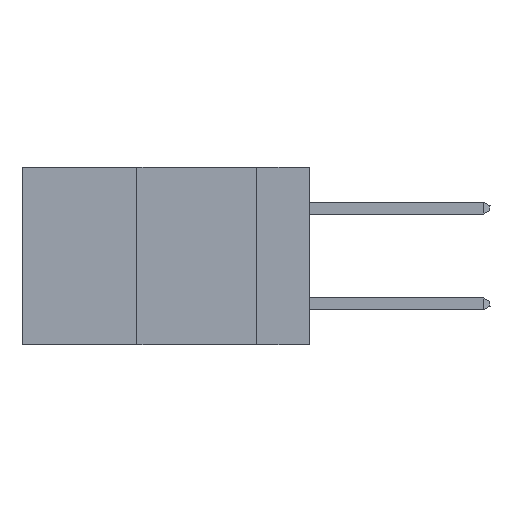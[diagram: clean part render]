
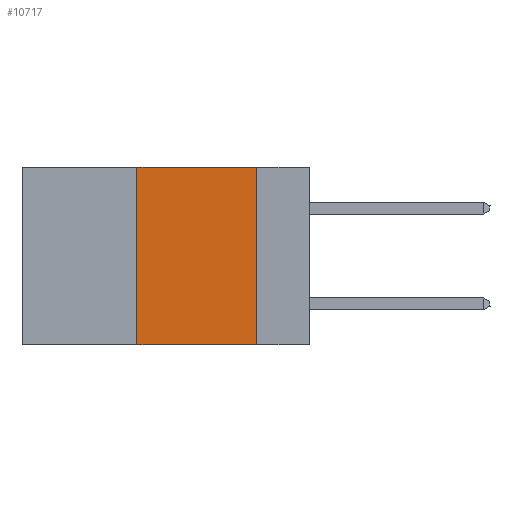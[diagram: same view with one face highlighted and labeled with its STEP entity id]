
A CAD part, left-side view. The second image highlights one B-rep face of the part: STEP entity #10717.
In plain terms, the highlighted planar face has unit normal (-1, 0, 0).
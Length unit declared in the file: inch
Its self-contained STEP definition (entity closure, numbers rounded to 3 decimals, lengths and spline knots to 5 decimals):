
#1146 = CARTESIAN_POINT ( 'NONE',  ( 0., 0.11, 0. ) ) ;
#1238 = VERTEX_POINT ( 'NONE', #8673 ) ;
#1321 = CARTESIAN_POINT ( 'NONE',  ( 0., 0.6, -0.37 ) ) ;
#1409 = VERTEX_POINT ( 'NONE', #10183 ) ;
#2096 = DIRECTION ( 'NONE',  ( 1., 0., 0. ) ) ;
#2197 = CARTESIAN_POINT ( 'NONE',  ( 0., 0.36, 0. ) ) ;
#2538 = ORIENTED_EDGE ( 'NONE', *, *, #3859, .F. ) ;
#2765 = FACE_OUTER_BOUND ( 'NONE', #9838, .T. ) ;
#2970 = CARTESIAN_POINT ( 'NONE',  ( 0., 0.6, 0. ) ) ;
#3279 = DIRECTION ( 'NONE',  ( 0., -1., 0. ) ) ;
#3540 = CARTESIAN_POINT ( 'NONE',  ( 0., 0.36, -0.37 ) ) ;
#3859 = EDGE_CURVE ( 'NONE', #5016, #6405, #11107, .T. ) ;
#4099 = ORIENTED_EDGE ( 'NONE', *, *, #12508, .T. ) ;
#4208 = DIRECTION ( 'NONE',  ( 0., 0., -1. ) ) ;
#4280 = LINE ( 'NONE', #1321, #11281 ) ;
#4393 = VECTOR ( 'NONE', #7071, 39.37008 ) ;
#4501 = EDGE_CURVE ( 'NONE', #6405, #1409, #8302, .T. ) ;
#4865 = VECTOR ( 'NONE', #5675, 39.37008 ) ;
#5016 = VERTEX_POINT ( 'NONE', #3540 ) ;
#5675 = DIRECTION ( 'NONE',  ( 0., 0., 1. ) ) ;
#6405 = VERTEX_POINT ( 'NONE', #2197 ) ;
#7071 = DIRECTION ( 'NONE',  ( 0., -1., 0. ) ) ;
#7522 = LINE ( 'NONE', #1146, #12227 ) ;
#7908 = DIRECTION ( 'NONE',  ( 0., 0., -1. ) ) ;
#8046 = PLANE ( 'NONE',  #8384 ) ;
#8076 = CARTESIAN_POINT ( 'NONE',  ( 0., 0.6, 0. ) ) ;
#8287 = ORIENTED_EDGE ( 'NONE', *, *, #12796, .F. ) ;
#8302 = LINE ( 'NONE', #8076, #4393 ) ;
#8384 = AXIS2_PLACEMENT_3D ( 'NONE', #2970, #2096, #7908 ) ;
#8673 = CARTESIAN_POINT ( 'NONE',  ( 0., 0.11, -0.37 ) ) ;
#9650 = CARTESIAN_POINT ( 'NONE',  ( 0., 0.36, 0. ) ) ;
#9838 = EDGE_LOOP ( 'NONE', ( #8287, #11392, #2538, #4099 ) ) ;
#10183 = CARTESIAN_POINT ( 'NONE',  ( 0., 0.11, 0. ) ) ;
#10717 = ADVANCED_FACE ( 'NONE', ( #2765 ), #8046, .F. ) ;
#11107 = LINE ( 'NONE', #9650, #4865 ) ;
#11281 = VECTOR ( 'NONE', #3279, 39.37008 ) ;
#11392 = ORIENTED_EDGE ( 'NONE', *, *, #4501, .F. ) ;
#12227 = VECTOR ( 'NONE', #4208, 39.37008 ) ;
#12508 = EDGE_CURVE ( 'NONE', #5016, #1238, #4280, .T. ) ;
#12796 = EDGE_CURVE ( 'NONE', #1409, #1238, #7522, .T. ) ;
